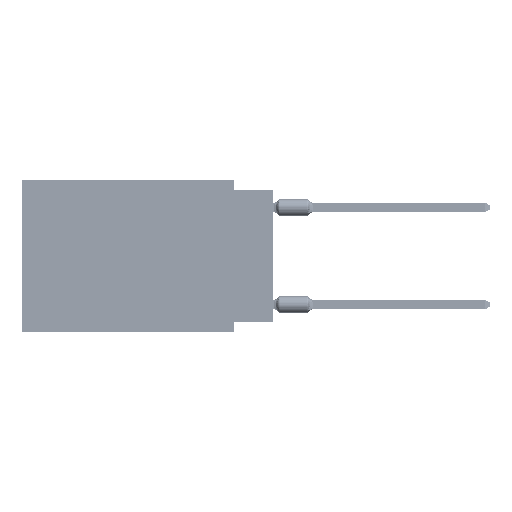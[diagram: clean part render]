
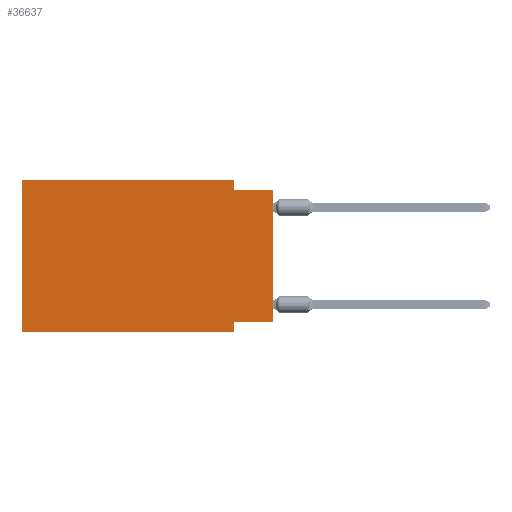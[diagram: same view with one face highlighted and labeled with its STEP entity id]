
A CAD part, left-side view. The second image highlights one B-rep face of the part: STEP entity #36637.
In plain terms, the highlighted planar face has unit normal (-1, 0, 0).
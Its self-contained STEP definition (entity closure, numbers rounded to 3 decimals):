
#1434 = DIRECTION ( 'NONE',  ( 0., -1., 0. ) ) ;
#2201 = VECTOR ( 'NONE', #23583, 1000. ) ;
#3794 = VECTOR ( 'NONE', #32397, 1000. ) ;
#4609 = ORIENTED_EDGE ( 'NONE', *, *, #73458, .F. ) ;
#6204 = EDGE_CURVE ( 'NONE', #11032, #18557, #60644, .T. ) ;
#6830 = FACE_OUTER_BOUND ( 'NONE', #7886, .T. ) ;
#7203 = EDGE_CURVE ( 'NONE', #34228, #13500, #18183, .T. ) ;
#7261 = LINE ( 'NONE', #57881, #3794 ) ;
#7886 = EDGE_LOOP ( 'NONE', ( #71666, #25204, #71697, #18873, #4609, #59792, #49091, #32734 ) ) ;
#8002 = PLANE ( 'NONE',  #24832 ) ;
#9293 = EDGE_CURVE ( 'NONE', #52432, #59678, #7261, .T. ) ;
#10248 = DIRECTION ( 'NONE',  ( 0., 0., 1. ) ) ;
#11032 = VERTEX_POINT ( 'NONE', #32719 ) ;
#12988 = VERTEX_POINT ( 'NONE', #14330 ) ;
#13500 = VERTEX_POINT ( 'NONE', #32987 ) ;
#14330 = CARTESIAN_POINT ( 'NONE',  ( 0., 16.383, -9.906 ) ) ;
#16459 = VECTOR ( 'NONE', #59285, 1000. ) ;
#18183 = LINE ( 'NONE', #32030, #74862 ) ;
#18557 = VERTEX_POINT ( 'NONE', #19348 ) ;
#18603 = CARTESIAN_POINT ( 'NONE',  ( 0., 0., -0.635 ) ) ;
#18873 = ORIENTED_EDGE ( 'NONE', *, *, #7203, .F. ) ;
#19348 = CARTESIAN_POINT ( 'NONE',  ( 0., 2.54, -9.906 ) ) ;
#23583 = DIRECTION ( 'NONE',  ( 0., 0., -1. ) ) ;
#24832 = AXIS2_PLACEMENT_3D ( 'NONE', #35703, #29717, #55911 ) ;
#25204 = ORIENTED_EDGE ( 'NONE', *, *, #78570, .F. ) ;
#27050 = EDGE_CURVE ( 'NONE', #12988, #18557, #78419, .T. ) ;
#28433 = LINE ( 'NONE', #77449, #63249 ) ;
#29447 = CARTESIAN_POINT ( 'NONE',  ( 0., 16.383, 0. ) ) ;
#29717 = DIRECTION ( 'NONE',  ( 1., 0., 0. ) ) ;
#30095 = LINE ( 'NONE', #60771, #63496 ) ;
#31020 = VECTOR ( 'NONE', #1434, 1000. ) ;
#32030 = CARTESIAN_POINT ( 'NONE',  ( 0., 16.383, 0. ) ) ;
#32143 = LINE ( 'NONE', #18603, #31020 ) ;
#32397 = DIRECTION ( 'NONE',  ( 0., 0., 1. ) ) ;
#32719 = CARTESIAN_POINT ( 'NONE',  ( 0., 2.54, -9.271 ) ) ;
#32734 = ORIENTED_EDGE ( 'NONE', *, *, #55385, .F. ) ;
#32987 = CARTESIAN_POINT ( 'NONE',  ( 0., 2.54, 0. ) ) ;
#33974 = VERTEX_POINT ( 'NONE', #62179 ) ;
#34228 = VERTEX_POINT ( 'NONE', #29447 ) ;
#35703 = CARTESIAN_POINT ( 'NONE',  ( 0., 16.383, 0. ) ) ;
#36637 = ADVANCED_FACE ( 'NONE', ( #6830 ), #8002, .F. ) ;
#38019 = DIRECTION ( 'NONE',  ( 0., -1., 0. ) ) ;
#44020 = DIRECTION ( 'NONE',  ( 0., 1., 0. ) ) ;
#49091 = ORIENTED_EDGE ( 'NONE', *, *, #6204, .F. ) ;
#52432 = VERTEX_POINT ( 'NONE', #75254 ) ;
#54278 = CARTESIAN_POINT ( 'NONE',  ( 0., 2.54, -9.906 ) ) ;
#55385 = EDGE_CURVE ( 'NONE', #52432, #11032, #30095, .T. ) ;
#55911 = DIRECTION ( 'NONE',  ( 0., 0., -1. ) ) ;
#57385 = CARTESIAN_POINT ( 'NONE',  ( 0., 0., -0.635 ) ) ;
#57881 = CARTESIAN_POINT ( 'NONE',  ( 0., 0., 0. ) ) ;
#59285 = DIRECTION ( 'NONE',  ( 0., -1., 0. ) ) ;
#59533 = VECTOR ( 'NONE', #10248, 1000. ) ;
#59678 = VERTEX_POINT ( 'NONE', #57385 ) ;
#59792 = ORIENTED_EDGE ( 'NONE', *, *, #27050, .T. ) ;
#60644 = LINE ( 'NONE', #54278, #2201 ) ;
#60771 = CARTESIAN_POINT ( 'NONE',  ( 0., 0., -9.271 ) ) ;
#62179 = CARTESIAN_POINT ( 'NONE',  ( 0., 2.54, -0.635 ) ) ;
#63249 = VECTOR ( 'NONE', #71856, 1000. ) ;
#63496 = VECTOR ( 'NONE', #44020, 1000. ) ;
#70305 = EDGE_CURVE ( 'NONE', #13500, #33974, #28433, .T. ) ;
#70470 = LINE ( 'NONE', #75282, #59533 ) ;
#71666 = ORIENTED_EDGE ( 'NONE', *, *, #9293, .T. ) ;
#71697 = ORIENTED_EDGE ( 'NONE', *, *, #70305, .F. ) ;
#71856 = DIRECTION ( 'NONE',  ( 0., 0., -1. ) ) ;
#73458 = EDGE_CURVE ( 'NONE', #12988, #34228, #70470, .T. ) ;
#74862 = VECTOR ( 'NONE', #38019, 1000. ) ;
#75254 = CARTESIAN_POINT ( 'NONE',  ( 0., 0., -9.271 ) ) ;
#75282 = CARTESIAN_POINT ( 'NONE',  ( 0., 16.383, 0. ) ) ;
#77449 = CARTESIAN_POINT ( 'NONE',  ( 0., 2.54, 0. ) ) ;
#77628 = CARTESIAN_POINT ( 'NONE',  ( 0., 16.383, -9.906 ) ) ;
#78419 = LINE ( 'NONE', #77628, #16459 ) ;
#78570 = EDGE_CURVE ( 'NONE', #33974, #59678, #32143, .T. ) ;
